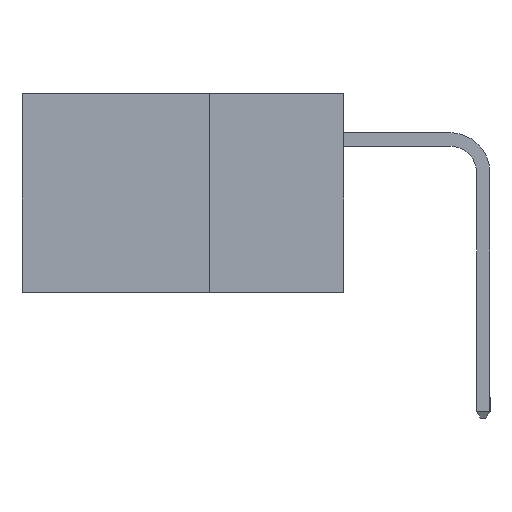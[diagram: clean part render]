
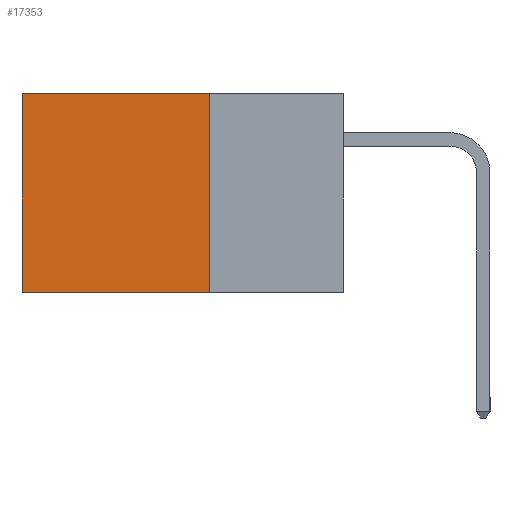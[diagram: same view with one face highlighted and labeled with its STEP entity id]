
A CAD part, left-side view. The second image highlights one B-rep face of the part: STEP entity #17353.
In plain terms, the highlighted planar face has unit normal (-1, 0, 0).
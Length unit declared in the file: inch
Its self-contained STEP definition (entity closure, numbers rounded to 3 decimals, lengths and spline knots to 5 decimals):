
#315 = DIRECTION ( 'NONE',  ( 0., 0., -1. ) ) ;
#563 = EDGE_CURVE ( 'NONE', #10410, #12110, #7059, .T. ) ;
#700 = DIRECTION ( 'NONE',  ( 0., 0., -1. ) ) ;
#804 = CARTESIAN_POINT ( 'NONE',  ( 0.2615, 0.25, 0. ) ) ;
#896 = CARTESIAN_POINT ( 'NONE',  ( 0.2615, 0.25, -0.37 ) ) ;
#1763 = ORIENTED_EDGE ( 'NONE', *, *, #18260, .F. ) ;
#1989 = VERTEX_POINT ( 'NONE', #16812 ) ;
#2661 = DIRECTION ( 'NONE',  ( 0., 1., 0. ) ) ;
#2963 = CARTESIAN_POINT ( 'NONE',  ( 0.2615, 0.6, 0. ) ) ;
#3281 = CARTESIAN_POINT ( 'NONE',  ( 0.2615, 0.6, -0.37 ) ) ;
#3357 = ORIENTED_EDGE ( 'NONE', *, *, #16655, .T. ) ;
#3488 = LINE ( 'NONE', #896, #22176 ) ;
#4678 = CARTESIAN_POINT ( 'NONE',  ( 0.2615, 0.25, -0.37 ) ) ;
#4958 = LINE ( 'NONE', #16855, #21983 ) ;
#6499 = PLANE ( 'NONE',  #22181 ) ;
#7059 = LINE ( 'NONE', #3281, #11268 ) ;
#7726 = EDGE_CURVE ( 'NONE', #19610, #1989, #3488, .T. ) ;
#8321 = DIRECTION ( 'NONE',  ( 0., 0., -1. ) ) ;
#9146 = ORIENTED_EDGE ( 'NONE', *, *, #563, .T. ) ;
#9892 = DIRECTION ( 'NONE',  ( 0., 1., 0. ) ) ;
#10410 = VERTEX_POINT ( 'NONE', #2963 ) ;
#11268 = VECTOR ( 'NONE', #700, 39.37008 ) ;
#12110 = VERTEX_POINT ( 'NONE', #12981 ) ;
#12914 = ORIENTED_EDGE ( 'NONE', *, *, #7726, .F. ) ;
#12981 = CARTESIAN_POINT ( 'NONE',  ( 0.2615, 0.6, -0.37 ) ) ;
#13431 = EDGE_LOOP ( 'NONE', ( #9146, #1763, #12914, #3357 ) ) ;
#14834 = LINE ( 'NONE', #18627, #22328 ) ;
#16655 = EDGE_CURVE ( 'NONE', #19610, #10410, #4958, .T. ) ;
#16812 = CARTESIAN_POINT ( 'NONE',  ( 0.2615, 0.25, -0.37 ) ) ;
#16855 = CARTESIAN_POINT ( 'NONE',  ( 0.2615, 0.25, 0. ) ) ;
#17353 = ADVANCED_FACE ( 'NONE', ( #20642 ), #6499, .F. ) ;
#18260 = EDGE_CURVE ( 'NONE', #1989, #12110, #14834, .T. ) ;
#18627 = CARTESIAN_POINT ( 'NONE',  ( 0.2615, 0.25, -0.37 ) ) ;
#19610 = VERTEX_POINT ( 'NONE', #804 ) ;
#20642 = FACE_OUTER_BOUND ( 'NONE', #13431, .T. ) ;
#21983 = VECTOR ( 'NONE', #2661, 39.37008 ) ;
#22176 = VECTOR ( 'NONE', #315, 39.37008 ) ;
#22177 = DIRECTION ( 'NONE',  ( 1., 0., 0. ) ) ;
#22181 = AXIS2_PLACEMENT_3D ( 'NONE', #4678, #22177, #8321 ) ;
#22328 = VECTOR ( 'NONE', #9892, 39.37008 ) ;
